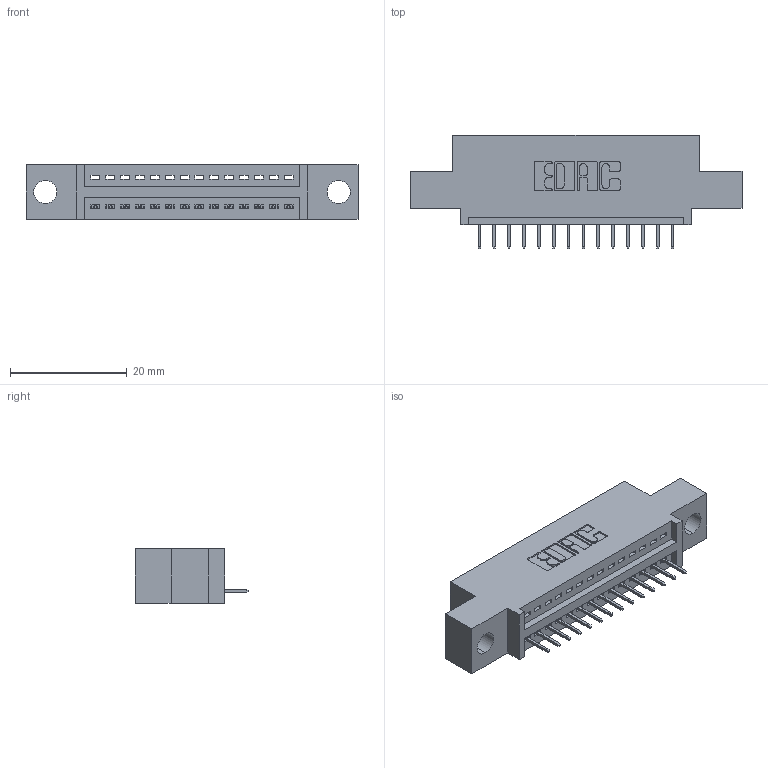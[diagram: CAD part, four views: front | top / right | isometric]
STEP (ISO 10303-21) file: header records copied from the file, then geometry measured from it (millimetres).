
FILE_DESCRIPTION (( 'STEP AP203' ), '1' );
FILE_NAME ('345-014-524-404.STEP', '2021-05-26T14:11:53', ( '' ), ( '' ), 'SwSTEP 2.0', 'SolidWorks 2020', '' );
FILE_SCHEMA (( 'CONFIG_CONTROL_DESIGN' ));
Length unit declared in the file: inch
Products named in the file (3): 345-014-524-404; 345-292-001_345-293-124; 345 Part_0.110 Offset - 0.156 Dia-TI
Assembly tree (15 placements, depth 2):
  345-014-524-404
    345 Part_0.110 Offset - 0.156 Dia-TI
    345-292-001_345-293-124  x14
Bounding box: 56.77 x 19.35 x 9.4 mm (x, y, z)
Volume: 4928 mm3; surface area: 5915.8 mm2
Topology: 15 solids, 15 shells, 1012 faces, 2909 edges, 1882 vertices
Faces by surface type: plane 742, cylinder 270
Entity records: 14931 total; most frequent: CARTESIAN_POINT 2596, ORIENTED_EDGE 2542, DIRECTION 2307, EDGE_CURVE 1271, VECTOR 1087, LINE 1087, VERTEX_POINT 842, AXIS2_PLACEMENT_3D 610
